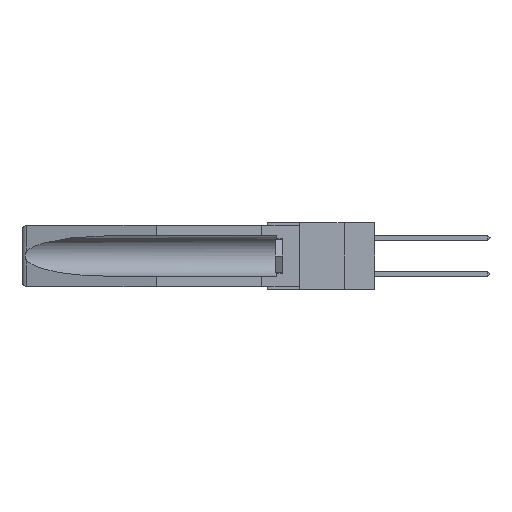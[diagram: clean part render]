
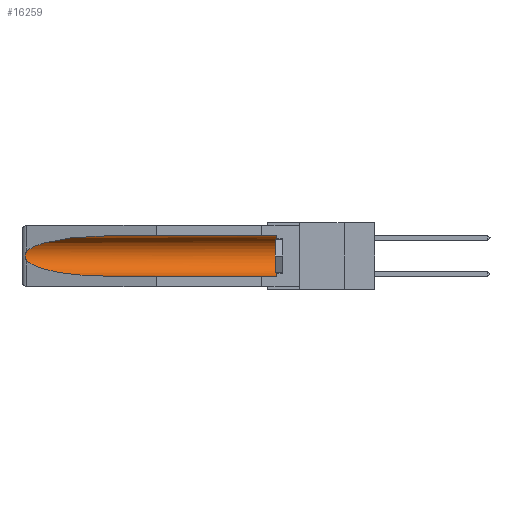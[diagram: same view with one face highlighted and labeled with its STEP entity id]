
A CAD part, left-side view. The second image highlights one B-rep face of the part: STEP entity #16259.
In plain terms, the highlighted cylindrical face has radius 2.857 mm (diameter 5.715 mm), a partial arc.
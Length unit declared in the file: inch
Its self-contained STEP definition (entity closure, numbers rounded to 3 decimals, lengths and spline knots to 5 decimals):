
#195 = CARTESIAN_POINT ( 'NONE',  ( 0.155, 1.07973, -0.284 ) ) ;
#709 = LINE ( 'NONE', #818, #20621 ) ;
#818 = CARTESIAN_POINT ( 'NONE',  ( 0.155, -0.30754, -0.059 ) ) ;
#1258 = VERTEX_POINT ( 'NONE', #8843 ) ;
#2774 = ORIENTED_EDGE ( 'NONE', *, *, #23385, .T. ) ;
#2852 = CARTESIAN_POINT ( 'NONE',  ( 0.21114, 1.30732, -0.059 ) ) ;
#5243 = CARTESIAN_POINT ( 'NONE',  ( 0.26597, 1.52961, -0.15275 ) ) ;
#5442 = CARTESIAN_POINT ( 'NONE',  ( 0.2675, 1.53308, -0.16763 ) ) ;
#6357 = VECTOR ( 'NONE', #19500, 39.37008 ) ;
#6802 = EDGE_LOOP ( 'NONE', ( #24757, #21348, #11761, #23214, #2774, #8737 ) ) ;
#7384 = CARTESIAN_POINT ( 'NONE',  ( 0.26537, 1.52718, -0.19328 ) ) ;
#7571 = CARTESIAN_POINT ( 'NONE',  ( 0.26537, 1.52718, -0.14972 ) ) ;
#8737 = ORIENTED_EDGE ( 'NONE', *, *, #10272, .T. ) ;
#8843 = CARTESIAN_POINT ( 'NONE',  ( 0.26537, 1.52718, -0.19328 ) ) ;
#9944 = CARTESIAN_POINT ( 'NONE',  ( 0.25451, 1.48313, -0.09465 ) ) ;
#10048 = B_SPLINE_CURVE_WITH_KNOTS ( 'NONE', 3,
 ( #7571, #5243, #12323, #23856, #5442, #21520, #26114, #16787, #21619, #7384 ),
 .UNSPECIFIED., .F., .F.,
 ( 4, 2, 2, 2, 4 ),
 ( 0., 0.00029, 0.00058, 0.00087, 0.00117 ),
 .UNSPECIFIED. ) ;
#10272 = EDGE_CURVE ( 'NONE', #14135, #29892, #709, .T. ) ;
#10287 = DIRECTION ( 'NONE',  ( 0., 1., 0. ) ) ;
#11399 = DIRECTION ( 'NONE',  ( 0., 0., 1. ) ) ;
#11702 = AXIS2_PLACEMENT_3D ( 'NONE', #22793, #29728, #11399 ) ;
#11761 = ORIENTED_EDGE ( 'NONE', *, *, #21970, .T. ) ;
#12323 = CARTESIAN_POINT ( 'NONE',  ( 0.26654, 1.53092, -0.15636 ) ) ;
#12559 = CARTESIAN_POINT ( 'NONE',  ( 0.25451, 1.48313, -0.24835 ) ) ;
#12586 = CARTESIAN_POINT ( 'NONE',  ( 0.155, -0.30754, -0.1715 ) ) ;
#14135 = VERTEX_POINT ( 'NONE', #27381 ) ;
#14811 = CARTESIAN_POINT ( 'NONE',  ( 0.155, 1.07973, -0.284 ) ) ;
#15425 =( BOUNDED_CURVE ( )  B_SPLINE_CURVE ( 3, ( #21453, #2852, #9944, #26456 ),
 .UNSPECIFIED., .F., .F. ) 
 B_SPLINE_CURVE_WITH_KNOTS ( ( 4, 4 ),
 ( 4.71239, 6.08839 ),
 .UNSPECIFIED. ) 
 CURVE ( )  GEOMETRIC_REPRESENTATION_ITEM ( )  RATIONAL_B_SPLINE_CURVE ( ( 1., 0.848, 0.848, 1. ) ) 
 REPRESENTATION_ITEM ( '' )  );
#15800 = CARTESIAN_POINT ( 'NONE',  ( 0.155, 1.07973, -0.059 ) ) ;
#16052 = VERTEX_POINT ( 'NONE', #195 ) ;
#16259 = ADVANCED_FACE ( 'NONE', ( #21952 ), #24140, .F. ) ;
#16437 = AXIS2_PLACEMENT_3D ( 'NONE', #12586, #10287, #23842 ) ;
#16787 = CARTESIAN_POINT ( 'NONE',  ( 0.26655, 1.53094, -0.18657 ) ) ;
#17342 = EDGE_CURVE ( 'NONE', #21436, #1258, #10048, .T. ) ;
#19040 = EDGE_CURVE ( 'NONE', #29892, #21436, #15425, .T. ) ;
#19500 = DIRECTION ( 'NONE',  ( 0., 1., 0. ) ) ;
#20621 = VECTOR ( 'NONE', #21472, 39.37008 ) ;
#20962 = VERTEX_POINT ( 'NONE', #26791 ) ;
#21274 = CARTESIAN_POINT ( 'NONE',  ( 0.21114, 1.30732, -0.284 ) ) ;
#21348 = ORIENTED_EDGE ( 'NONE', *, *, #17342, .T. ) ;
#21436 = VERTEX_POINT ( 'NONE', #22340 ) ;
#21453 = CARTESIAN_POINT ( 'NONE',  ( 0.155, 1.07973, -0.059 ) ) ;
#21472 = DIRECTION ( 'NONE',  ( 0., 1., 0. ) ) ;
#21520 = CARTESIAN_POINT ( 'NONE',  ( 0.2675, 1.53308, -0.17534 ) ) ;
#21619 = CARTESIAN_POINT ( 'NONE',  ( 0.26597, 1.5296, -0.19026 ) ) ;
#21935 = CARTESIAN_POINT ( 'NONE',  ( 0.155, -0.30754, -0.284 ) ) ;
#21952 = FACE_OUTER_BOUND ( 'NONE', #6802, .T. ) ;
#21970 = EDGE_CURVE ( 'NONE', #1258, #16052, #26216, .T. ) ;
#22340 = CARTESIAN_POINT ( 'NONE',  ( 0.26537, 1.52718, -0.14972 ) ) ;
#22668 = CIRCLE ( 'NONE', #11702, 0.1125 ) ;
#22793 = CARTESIAN_POINT ( 'NONE',  ( 0.155, 0.126, -0.1715 ) ) ;
#23214 = ORIENTED_EDGE ( 'NONE', *, *, #26264, .F. ) ;
#23385 = EDGE_CURVE ( 'NONE', #20962, #14135, #22668, .T. ) ;
#23842 = DIRECTION ( 'NONE',  ( 0., 0., 1. ) ) ;
#23856 = CARTESIAN_POINT ( 'NONE',  ( 0.2673, 1.5327, -0.16383 ) ) ;
#24140 = CYLINDRICAL_SURFACE ( 'NONE', #16437, 0.1125 ) ;
#24757 = ORIENTED_EDGE ( 'NONE', *, *, #19040, .T. ) ;
#26114 = CARTESIAN_POINT ( 'NONE',  ( 0.2673, 1.53269, -0.17917 ) ) ;
#26216 =( BOUNDED_CURVE ( )  B_SPLINE_CURVE ( 3, ( #28170, #12559, #21274, #14811 ),
 .UNSPECIFIED., .F., .F. ) 
 B_SPLINE_CURVE_WITH_KNOTS ( ( 4, 4 ),
 ( 0.1948, 1.5708 ),
 .UNSPECIFIED. ) 
 CURVE ( )  GEOMETRIC_REPRESENTATION_ITEM ( )  RATIONAL_B_SPLINE_CURVE ( ( 1., 0.848, 0.848, 1. ) ) 
 REPRESENTATION_ITEM ( '' )  );
#26264 = EDGE_CURVE ( 'NONE', #20962, #16052, #28441, .T. ) ;
#26456 = CARTESIAN_POINT ( 'NONE',  ( 0.26537, 1.52718, -0.14972 ) ) ;
#26791 = CARTESIAN_POINT ( 'NONE',  ( 0.155, 0.126, -0.284 ) ) ;
#27381 = CARTESIAN_POINT ( 'NONE',  ( 0.155, 0.126, -0.059 ) ) ;
#28170 = CARTESIAN_POINT ( 'NONE',  ( 0.26537, 1.52718, -0.19328 ) ) ;
#28441 = LINE ( 'NONE', #21935, #6357 ) ;
#29728 = DIRECTION ( 'NONE',  ( 0., -1., 0. ) ) ;
#29892 = VERTEX_POINT ( 'NONE', #15800 ) ;
